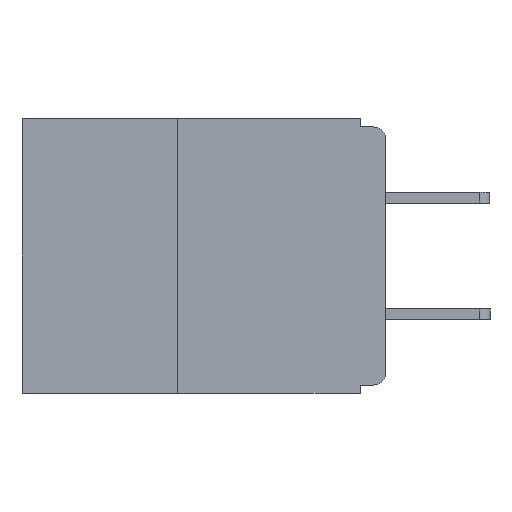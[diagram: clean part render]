
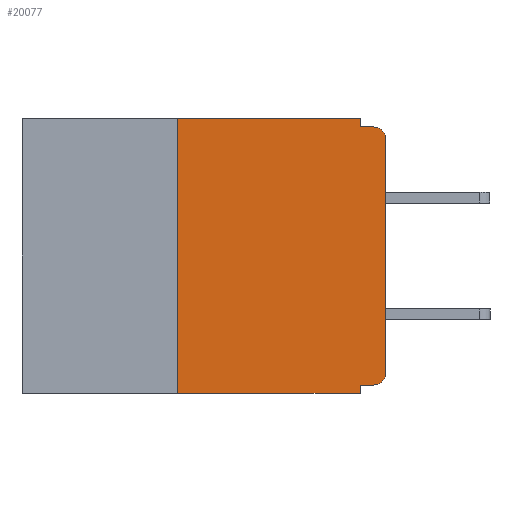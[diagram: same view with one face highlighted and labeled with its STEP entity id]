
A CAD part, left-side view. The second image highlights one B-rep face of the part: STEP entity #20077.
In plain terms, the highlighted planar face has unit normal (-1, 0, 0).
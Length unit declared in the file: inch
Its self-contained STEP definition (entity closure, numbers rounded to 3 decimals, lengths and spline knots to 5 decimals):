
#128 = ORIENTED_EDGE ( 'NONE', *, *, #32739, .F. ) ;
#1276 = ORIENTED_EDGE ( 'NONE', *, *, #31074, .F. ) ;
#2262 = PLANE ( 'NONE',  #24295 ) ;
#2316 = ORIENTED_EDGE ( 'NONE', *, *, #16049, .T. ) ;
#2416 = VERTEX_POINT ( 'NONE', #13154 ) ;
#2454 = VECTOR ( 'NONE', #16689, 39.37008 ) ;
#2561 = VECTOR ( 'NONE', #14648, 39.37008 ) ;
#2952 = CARTESIAN_POINT ( 'NONE',  ( 0., 0., 0. ) ) ;
#4945 = CARTESIAN_POINT ( 'NONE',  ( 0., 0.437, 0. ) ) ;
#4995 = CARTESIAN_POINT ( 'NONE',  ( 0., 0., -0.025 ) ) ;
#5340 = LINE ( 'NONE', #20837, #31344 ) ;
#6010 = ORIENTED_EDGE ( 'NONE', *, *, #15597, .F. ) ;
#6261 = ORIENTED_EDGE ( 'NONE', *, *, #8520, .T. ) ;
#6337 = CARTESIAN_POINT ( 'NONE',  ( 0., 0., -0.32 ) ) ;
#6965 = VECTOR ( 'NONE', #21484, 39.37008 ) ;
#7285 = DIRECTION ( 'NONE',  ( -1., 0., 0. ) ) ;
#7884 = VECTOR ( 'NONE', #25095, 39.37008 ) ;
#7931 = CARTESIAN_POINT ( 'NONE',  ( 0., 0.437, 0. ) ) ;
#7990 = VERTEX_POINT ( 'NONE', #28913 ) ;
#8253 = ORIENTED_EDGE ( 'NONE', *, *, #15542, .F. ) ;
#8410 = VERTEX_POINT ( 'NONE', #17724 ) ;
#8488 = CARTESIAN_POINT ( 'NONE',  ( 0., 0.031, 0. ) ) ;
#8520 = EDGE_CURVE ( 'NONE', #27280, #7990, #29184, .T. ) ;
#8647 = LINE ( 'NONE', #6337, #14834 ) ;
#8706 = LINE ( 'NONE', #12051, #7884 ) ;
#9458 = EDGE_LOOP ( 'NONE', ( #2316, #6261, #26118, #128, #11234, #1276, #14807, #8253, #6010, #13432 ) ) ;
#9463 = LINE ( 'NONE', #13958, #2454 ) ;
#9603 = EDGE_CURVE ( 'NONE', #31260, #7990, #17410, .T. ) ;
#10570 = DIRECTION ( 'NONE',  ( 0., -1., 0. ) ) ;
#11234 = ORIENTED_EDGE ( 'NONE', *, *, #13999, .F. ) ;
#12005 = CARTESIAN_POINT ( 'NONE',  ( 0., 0., -0.01 ) ) ;
#12051 = CARTESIAN_POINT ( 'NONE',  ( 0., 0.25, -0.33 ) ) ;
#12675 = LINE ( 'NONE', #8488, #25735 ) ;
#12915 = DIRECTION ( 'NONE',  ( 0., 0., -1. ) ) ;
#13020 = DIRECTION ( 'NONE',  ( -1., 0., 0. ) ) ;
#13154 = CARTESIAN_POINT ( 'NONE',  ( 0., 0.031, -0.33 ) ) ;
#13432 = ORIENTED_EDGE ( 'NONE', *, *, #24993, .T. ) ;
#13958 = CARTESIAN_POINT ( 'NONE',  ( 0., 0.031, -0.33 ) ) ;
#13999 = EDGE_CURVE ( 'NONE', #18957, #28970, #17845, .T. ) ;
#14648 = DIRECTION ( 'NONE',  ( 0., -1., 0. ) ) ;
#14797 = LINE ( 'NONE', #2952, #6965 ) ;
#14807 = ORIENTED_EDGE ( 'NONE', *, *, #26015, .T. ) ;
#14834 = VECTOR ( 'NONE', #22084, 39.37008 ) ;
#15501 = CARTESIAN_POINT ( 'NONE',  ( 0., 0.031, -0.01 ) ) ;
#15542 = EDGE_CURVE ( 'NONE', #23303, #2416, #9463, .T. ) ;
#15597 = EDGE_CURVE ( 'NONE', #17595, #23303, #8647, .T. ) ;
#16049 = EDGE_CURVE ( 'NONE', #8410, #27280, #14797, .T. ) ;
#16689 = DIRECTION ( 'NONE',  ( 0., 0., -1. ) ) ;
#16990 = VECTOR ( 'NONE', #10570, 39.37008 ) ;
#17410 = LINE ( 'NONE', #12005, #2561 ) ;
#17595 = VERTEX_POINT ( 'NONE', #28405 ) ;
#17724 = CARTESIAN_POINT ( 'NONE',  ( 0., 0., -0.305 ) ) ;
#17845 = LINE ( 'NONE', #7931, #16990 ) ;
#18116 = DIRECTION ( 'NONE',  ( 0., -1., 0. ) ) ;
#18957 = VERTEX_POINT ( 'NONE', #29329 ) ;
#20077 = ADVANCED_FACE ( 'NONE', ( #30841 ), #2262, .F. ) ;
#20099 = VERTEX_POINT ( 'NONE', #23434 ) ;
#20531 = AXIS2_PLACEMENT_3D ( 'NONE', #28539, #13020, #31072 ) ;
#20703 = AXIS2_PLACEMENT_3D ( 'NONE', #23025, #7285, #25616 ) ;
#20837 = CARTESIAN_POINT ( 'NONE',  ( 0., 0.437, -0.33 ) ) ;
#21484 = DIRECTION ( 'NONE',  ( 0., 0., 1. ) ) ;
#22084 = DIRECTION ( 'NONE',  ( 0., 1., 0. ) ) ;
#23025 = CARTESIAN_POINT ( 'NONE',  ( 0., 0.015, -0.305 ) ) ;
#23303 = VERTEX_POINT ( 'NONE', #23932 ) ;
#23434 = CARTESIAN_POINT ( 'NONE',  ( 0., 0.25, -0.33 ) ) ;
#23932 = CARTESIAN_POINT ( 'NONE',  ( 0., 0.031, -0.32 ) ) ;
#24295 = AXIS2_PLACEMENT_3D ( 'NONE', #4945, #28432, #12915 ) ;
#24993 = EDGE_CURVE ( 'NONE', #17595, #8410, #27349, .T. ) ;
#25095 = DIRECTION ( 'NONE',  ( 0., 0., 1. ) ) ;
#25616 = DIRECTION ( 'NONE',  ( 0., 0., -1. ) ) ;
#25735 = VECTOR ( 'NONE', #29302, 39.37008 ) ;
#26015 = EDGE_CURVE ( 'NONE', #20099, #2416, #5340, .T. ) ;
#26118 = ORIENTED_EDGE ( 'NONE', *, *, #9603, .F. ) ;
#27280 = VERTEX_POINT ( 'NONE', #4995 ) ;
#27349 = CIRCLE ( 'NONE', #20703, 0.015 ) ;
#28405 = CARTESIAN_POINT ( 'NONE',  ( 0., 0.015, -0.32 ) ) ;
#28432 = DIRECTION ( 'NONE',  ( 1., 0., 0. ) ) ;
#28539 = CARTESIAN_POINT ( 'NONE',  ( 0., 0.015, -0.025 ) ) ;
#28913 = CARTESIAN_POINT ( 'NONE',  ( 0., 0.015, -0.01 ) ) ;
#28970 = VERTEX_POINT ( 'NONE', #30527 ) ;
#29184 = CIRCLE ( 'NONE', #20531, 0.015 ) ;
#29302 = DIRECTION ( 'NONE',  ( 0., 0., -1. ) ) ;
#29329 = CARTESIAN_POINT ( 'NONE',  ( 0., 0.25, 0. ) ) ;
#30527 = CARTESIAN_POINT ( 'NONE',  ( 0., 0.031, 0. ) ) ;
#30841 = FACE_OUTER_BOUND ( 'NONE', #9458, .T. ) ;
#31072 = DIRECTION ( 'NONE',  ( 0., 0., -1. ) ) ;
#31074 = EDGE_CURVE ( 'NONE', #20099, #18957, #8706, .T. ) ;
#31260 = VERTEX_POINT ( 'NONE', #15501 ) ;
#31344 = VECTOR ( 'NONE', #18116, 39.37008 ) ;
#32739 = EDGE_CURVE ( 'NONE', #28970, #31260, #12675, .T. ) ;
